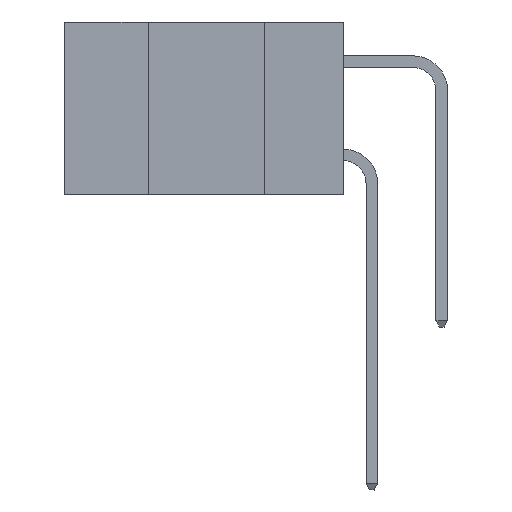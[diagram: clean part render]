
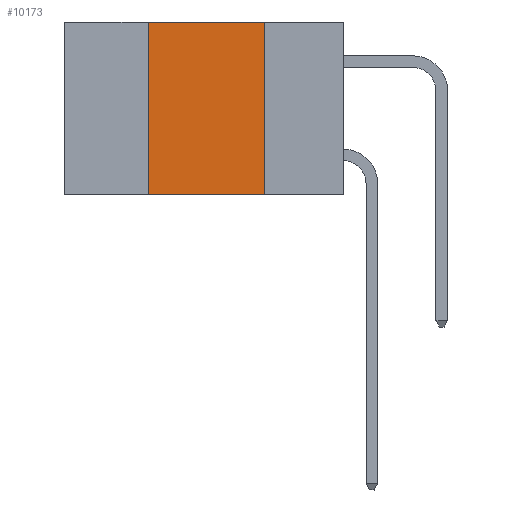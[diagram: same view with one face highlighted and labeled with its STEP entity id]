
A CAD part, left-side view. The second image highlights one B-rep face of the part: STEP entity #10173.
In plain terms, the highlighted planar face has unit normal (-1, 0, 0).
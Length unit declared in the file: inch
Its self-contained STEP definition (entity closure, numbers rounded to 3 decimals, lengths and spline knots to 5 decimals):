
#636 = LINE ( 'NONE', #13734, #11992 ) ;
#850 = ORIENTED_EDGE ( 'NONE', *, *, #14244, .F. ) ;
#5552 = VECTOR ( 'NONE', #5753, 39.37008 ) ;
#5753 = DIRECTION ( 'NONE',  ( 0., -1., 0. ) ) ;
#6149 = CARTESIAN_POINT ( 'NONE',  ( 0., 0.42, 0. ) ) ;
#6380 = PLANE ( 'NONE',  #7155 ) ;
#6827 = EDGE_CURVE ( 'NONE', #24002, #12279, #24627, .T. ) ;
#7155 = AXIS2_PLACEMENT_3D ( 'NONE', #15274, #8646, #24267 ) ;
#7751 = EDGE_CURVE ( 'NONE', #8493, #15448, #636, .T. ) ;
#8493 = VERTEX_POINT ( 'NONE', #27453 ) ;
#8646 = DIRECTION ( 'NONE',  ( 1., 0., 0. ) ) ;
#9292 = ORIENTED_EDGE ( 'NONE', *, *, #6827, .F. ) ;
#9701 = ORIENTED_EDGE ( 'NONE', *, *, #12478, .T. ) ;
#10173 = ADVANCED_FACE ( 'NONE', ( #10329 ), #6380, .F. ) ;
#10229 = VECTOR ( 'NONE', #20219, 39.37008 ) ;
#10329 = FACE_OUTER_BOUND ( 'NONE', #28843, .T. ) ;
#11992 = VECTOR ( 'NONE', #20480, 39.37008 ) ;
#12279 = VERTEX_POINT ( 'NONE', #6149 ) ;
#12478 = EDGE_CURVE ( 'NONE', #24002, #15448, #28025, .T. ) ;
#13402 = CARTESIAN_POINT ( 'NONE',  ( 0., 0.42, -0.37 ) ) ;
#13734 = CARTESIAN_POINT ( 'NONE',  ( 0., 0.17, -0.37 ) ) ;
#13926 = ORIENTED_EDGE ( 'NONE', *, *, #7751, .F. ) ;
#14244 = EDGE_CURVE ( 'NONE', #12279, #8493, #28621, .T. ) ;
#15274 = CARTESIAN_POINT ( 'NONE',  ( 0., 0.6, 0. ) ) ;
#15448 = VERTEX_POINT ( 'NONE', #19085 ) ;
#15727 = CARTESIAN_POINT ( 'NONE',  ( 0., 0.6, -0.37 ) ) ;
#16835 = CARTESIAN_POINT ( 'NONE',  ( 0., 0.42, -0.37 ) ) ;
#19085 = CARTESIAN_POINT ( 'NONE',  ( 0., 0.17, -0.37 ) ) ;
#20085 = VECTOR ( 'NONE', #29014, 39.37008 ) ;
#20219 = DIRECTION ( 'NONE',  ( 0., -1., 0. ) ) ;
#20480 = DIRECTION ( 'NONE',  ( 0., 0., -1. ) ) ;
#21382 = CARTESIAN_POINT ( 'NONE',  ( 0., 0.6, 0. ) ) ;
#24002 = VERTEX_POINT ( 'NONE', #16835 ) ;
#24267 = DIRECTION ( 'NONE',  ( 0., 0., -1. ) ) ;
#24627 = LINE ( 'NONE', #13402, #20085 ) ;
#27453 = CARTESIAN_POINT ( 'NONE',  ( 0., 0.17, 0. ) ) ;
#28025 = LINE ( 'NONE', #15727, #10229 ) ;
#28621 = LINE ( 'NONE', #21382, #5552 ) ;
#28843 = EDGE_LOOP ( 'NONE', ( #13926, #850, #9292, #9701 ) ) ;
#29014 = DIRECTION ( 'NONE',  ( 0., 0., 1. ) ) ;
